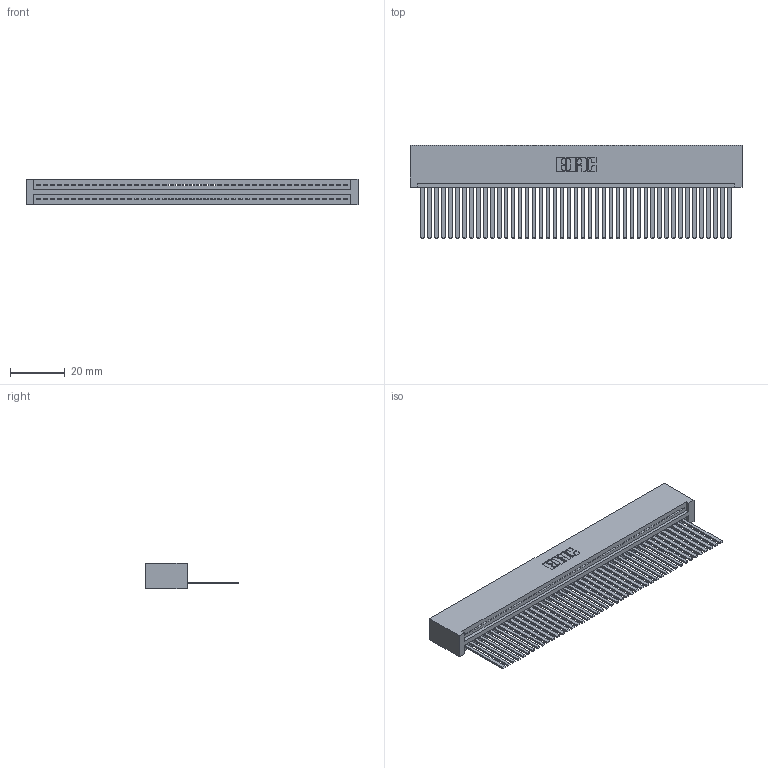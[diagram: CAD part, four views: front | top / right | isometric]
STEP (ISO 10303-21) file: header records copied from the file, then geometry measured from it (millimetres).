
FILE_DESCRIPTION (( 'STEP AP203' ), '1' );
FILE_NAME ('395-045-544-101.STEP', '2019-10-22T19:19:37', ( '' ), ( '' ), 'SwSTEP 2.0', 'SolidWorks 2016', '' );
FILE_SCHEMA (( 'CONFIG_CONTROL_DESIGN' ));
Length unit declared in the file: inch
Products named in the file (3): 395-045-544-101; 345-292-001_345-293-144; 345 Part_No Mounting Lugs
Assembly tree (46 placements, depth 2):
  395-045-544-101
    345 Part_No Mounting Lugs
    345-292-001_345-293-144  x45
Bounding box: 120.9 x 33.96 x 9.4 mm (x, y, z)
Volume: 12613.7 mm3; surface area: 18557.9 mm2
Topology: 46 solids, 46 shells, 2458 faces, 7427 edges, 4890 vertices
Faces by surface type: plane 1696, cylinder 762
Entity records: 33003 total; most frequent: CARTESIAN_POINT 5723, ORIENTED_EDGE 5702, DIRECTION 4985, EDGE_CURVE 2851, LINE 2551, VECTOR 2551, VERTEX_POINT 1898, AXIS2_PLACEMENT_3D 1217
